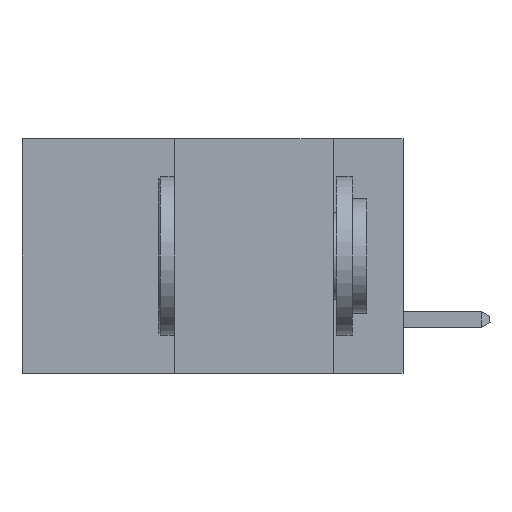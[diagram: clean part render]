
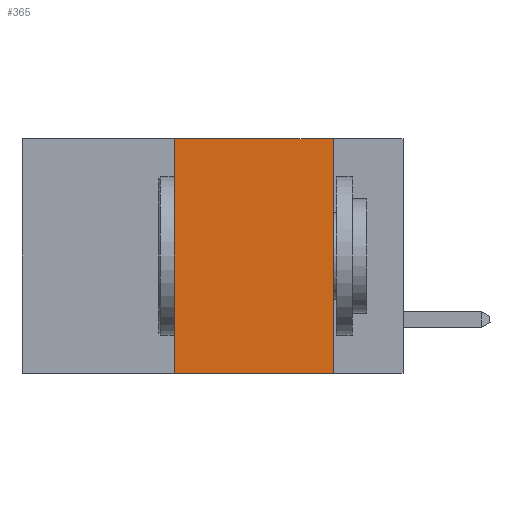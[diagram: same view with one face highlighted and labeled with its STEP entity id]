
A CAD part, left-side view. The second image highlights one B-rep face of the part: STEP entity #365.
In plain terms, the highlighted planar face has unit normal (-1, 0, 0).
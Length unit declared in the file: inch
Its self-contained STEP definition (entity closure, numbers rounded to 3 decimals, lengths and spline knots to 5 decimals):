
#335 = VERTEX_POINT ( 'NONE', #5477 ) ;
#365 = ADVANCED_FACE ( 'NONE', ( #5573 ), #540, .F. ) ;
#436 = CARTESIAN_POINT ( 'NONE',  ( 0., 0.6, 0. ) ) ;
#540 = PLANE ( 'NONE',  #7015 ) ;
#881 = VECTOR ( 'NONE', #6100, 39.37008 ) ;
#1172 = VECTOR ( 'NONE', #11723, 39.37008 ) ;
#1253 = DIRECTION ( 'NONE',  ( 0., -1., 0. ) ) ;
#1302 = VERTEX_POINT ( 'NONE', #5600 ) ;
#1329 = CARTESIAN_POINT ( 'NONE',  ( 0., 0.6, -0.37 ) ) ;
#1592 = ORIENTED_EDGE ( 'NONE', *, *, #1853, .F. ) ;
#1677 = LINE ( 'NONE', #1329, #8874 ) ;
#1771 = CARTESIAN_POINT ( 'NONE',  ( 0., 0.36, -0.37 ) ) ;
#1781 = CARTESIAN_POINT ( 'NONE',  ( 0., 0.36, 0. ) ) ;
#1853 = EDGE_CURVE ( 'NONE', #3611, #335, #12056, .T. ) ;
#2094 = CARTESIAN_POINT ( 'NONE',  ( 0., 0.36, 0. ) ) ;
#2562 = ORIENTED_EDGE ( 'NONE', *, *, #3660, .T. ) ;
#3175 = ORIENTED_EDGE ( 'NONE', *, *, #9465, .F. ) ;
#3211 = ORIENTED_EDGE ( 'NONE', *, *, #8232, .F. ) ;
#3611 = VERTEX_POINT ( 'NONE', #1781 ) ;
#3660 = EDGE_CURVE ( 'NONE', #11299, #1302, #1677, .T. ) ;
#5416 = EDGE_LOOP ( 'NONE', ( #3175, #1592, #3211, #2562 ) ) ;
#5477 = CARTESIAN_POINT ( 'NONE',  ( 0., 0.11, 0. ) ) ;
#5573 = FACE_OUTER_BOUND ( 'NONE', #5416, .T. ) ;
#5600 = CARTESIAN_POINT ( 'NONE',  ( 0., 0.11, -0.37 ) ) ;
#6100 = DIRECTION ( 'NONE',  ( 0., 0., 1. ) ) ;
#6544 = DIRECTION ( 'NONE',  ( 0., -1., 0. ) ) ;
#6571 = LINE ( 'NONE', #2094, #881 ) ;
#6631 = CARTESIAN_POINT ( 'NONE',  ( 0., 0.6, 0. ) ) ;
#7015 = AXIS2_PLACEMENT_3D ( 'NONE', #436, #7765, #8999 ) ;
#7765 = DIRECTION ( 'NONE',  ( 1., 0., 0. ) ) ;
#8232 = EDGE_CURVE ( 'NONE', #11299, #3611, #6571, .T. ) ;
#8874 = VECTOR ( 'NONE', #1253, 39.37008 ) ;
#8993 = LINE ( 'NONE', #9769, #1172 ) ;
#8999 = DIRECTION ( 'NONE',  ( 0., 0., -1. ) ) ;
#9465 = EDGE_CURVE ( 'NONE', #335, #1302, #8993, .T. ) ;
#9769 = CARTESIAN_POINT ( 'NONE',  ( 0., 0.11, 0. ) ) ;
#11299 = VERTEX_POINT ( 'NONE', #1771 ) ;
#11723 = DIRECTION ( 'NONE',  ( 0., 0., -1. ) ) ;
#12056 = LINE ( 'NONE', #6631, #12648 ) ;
#12648 = VECTOR ( 'NONE', #6544, 39.37008 ) ;
